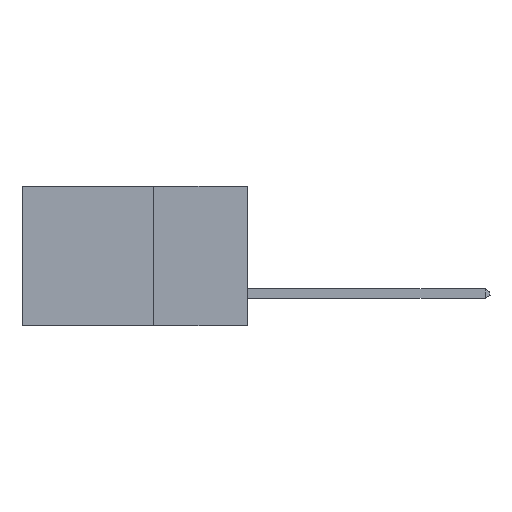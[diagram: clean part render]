
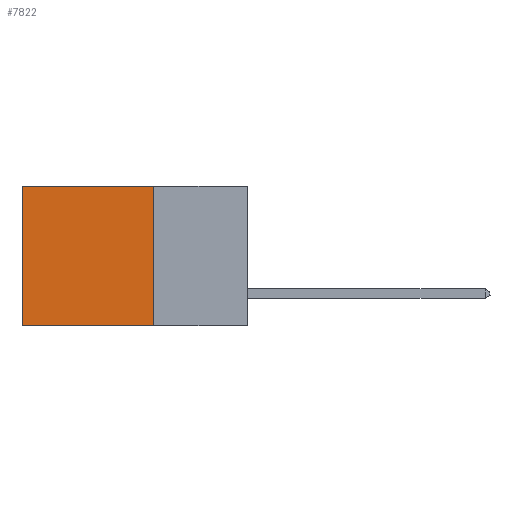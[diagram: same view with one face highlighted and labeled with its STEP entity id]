
A CAD part, left-side view. The second image highlights one B-rep face of the part: STEP entity #7822.
In plain terms, the highlighted planar face has unit normal (-1, 0, 0).
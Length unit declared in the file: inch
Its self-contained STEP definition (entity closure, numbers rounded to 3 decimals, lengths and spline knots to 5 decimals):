
#88 = VERTEX_POINT ( 'NONE', #7209 ) ;
#617 = ORIENTED_EDGE ( 'NONE', *, *, #31518, .F. ) ;
#1618 = VERTEX_POINT ( 'NONE', #26284 ) ;
#1694 = CARTESIAN_POINT ( 'NONE',  ( 0.298, 0.25, 0. ) ) ;
#1931 = CARTESIAN_POINT ( 'NONE',  ( 0.298, 0.6, 0. ) ) ;
#2040 = ORIENTED_EDGE ( 'NONE', *, *, #18472, .T. ) ;
#4864 = VECTOR ( 'NONE', #7897, 39.37008 ) ;
#6999 = DIRECTION ( 'NONE',  ( 0., 0., -1. ) ) ;
#7209 = CARTESIAN_POINT ( 'NONE',  ( 0.298, 0.25, -0.37 ) ) ;
#7822 = ADVANCED_FACE ( 'NONE', ( #25381 ), #16293, .F. ) ;
#7897 = DIRECTION ( 'NONE',  ( 0., 1., 0. ) ) ;
#8412 = DIRECTION ( 'NONE',  ( 0., 1., 0. ) ) ;
#9842 = CARTESIAN_POINT ( 'NONE',  ( 0.298, 0.6, -0.37 ) ) ;
#9891 = VERTEX_POINT ( 'NONE', #9842 ) ;
#12488 = LINE ( 'NONE', #18470, #13679 ) ;
#13285 = LINE ( 'NONE', #15498, #32048 ) ;
#13345 = VECTOR ( 'NONE', #6999, 39.37008 ) ;
#13679 = VECTOR ( 'NONE', #8412, 39.37008 ) ;
#15498 = CARTESIAN_POINT ( 'NONE',  ( 0.298, 0.25, 0. ) ) ;
#16293 = PLANE ( 'NONE',  #21774 ) ;
#17337 = EDGE_CURVE ( 'NONE', #24660, #9891, #25896, .T. ) ;
#18389 = CARTESIAN_POINT ( 'NONE',  ( 0.298, 0.6, 0. ) ) ;
#18470 = CARTESIAN_POINT ( 'NONE',  ( 0.298, 0.25, -0.37 ) ) ;
#18472 = EDGE_CURVE ( 'NONE', #1618, #24660, #29502, .T. ) ;
#20188 = EDGE_LOOP ( 'NONE', ( #29644, #617, #22930, #2040 ) ) ;
#21774 = AXIS2_PLACEMENT_3D ( 'NONE', #1694, #26383, #23981 ) ;
#22930 = ORIENTED_EDGE ( 'NONE', *, *, #31450, .F. ) ;
#23981 = DIRECTION ( 'NONE',  ( 0., 0., -1. ) ) ;
#24660 = VERTEX_POINT ( 'NONE', #18389 ) ;
#25381 = FACE_OUTER_BOUND ( 'NONE', #20188, .T. ) ;
#25896 = LINE ( 'NONE', #1931, #13345 ) ;
#26284 = CARTESIAN_POINT ( 'NONE',  ( 0.298, 0.25, 0. ) ) ;
#26383 = DIRECTION ( 'NONE',  ( 1., 0., 0. ) ) ;
#27655 = DIRECTION ( 'NONE',  ( 0., 0., -1. ) ) ;
#27905 = CARTESIAN_POINT ( 'NONE',  ( 0.298, 0.25, 0. ) ) ;
#29502 = LINE ( 'NONE', #27905, #4864 ) ;
#29644 = ORIENTED_EDGE ( 'NONE', *, *, #17337, .T. ) ;
#31450 = EDGE_CURVE ( 'NONE', #1618, #88, #13285, .T. ) ;
#31518 = EDGE_CURVE ( 'NONE', #88, #9891, #12488, .T. ) ;
#32048 = VECTOR ( 'NONE', #27655, 39.37008 ) ;
